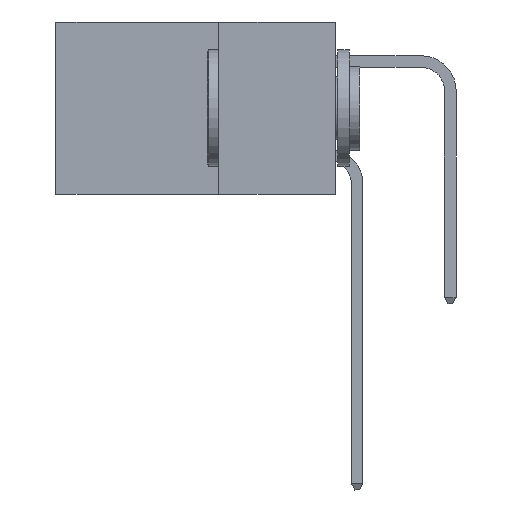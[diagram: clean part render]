
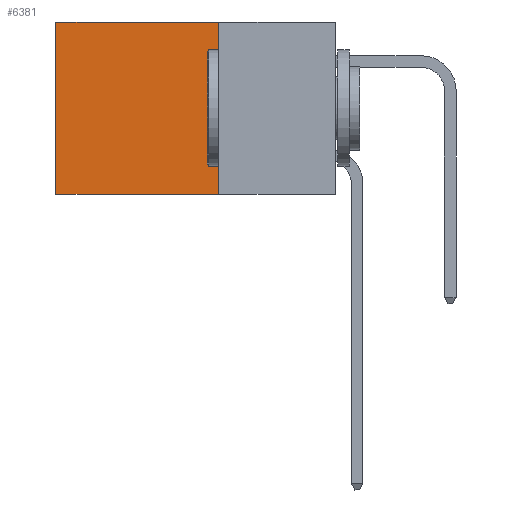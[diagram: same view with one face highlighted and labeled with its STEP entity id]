
A CAD part, left-side view. The second image highlights one B-rep face of the part: STEP entity #6381.
In plain terms, the highlighted planar face has unit normal (-1, 0, 0).
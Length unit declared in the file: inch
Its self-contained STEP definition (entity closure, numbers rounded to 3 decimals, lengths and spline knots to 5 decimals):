
#3 = CARTESIAN_POINT ( 'NONE',  ( 0.2875, 0.6, 0. ) ) ;
#42 = LINE ( 'NONE', #8670, #1972 ) ;
#457 = DIRECTION ( 'NONE',  ( 0., 1., 0. ) ) ;
#927 = ORIENTED_EDGE ( 'NONE', *, *, #6193, .F. ) ;
#1225 = LINE ( 'NONE', #3, #19461 ) ;
#1631 = VERTEX_POINT ( 'NONE', #9427 ) ;
#1972 = VECTOR ( 'NONE', #19196, 39.37008 ) ;
#2108 = LINE ( 'NONE', #10840, #22839 ) ;
#2180 = EDGE_CURVE ( 'NONE', #3280, #7720, #42, .T. ) ;
#3280 = VERTEX_POINT ( 'NONE', #22002 ) ;
#4042 = DIRECTION ( 'NONE',  ( 0., 0., -1. ) ) ;
#4323 = CARTESIAN_POINT ( 'NONE',  ( 0.2875, 0.25, -0.37 ) ) ;
#5308 = DIRECTION ( 'NONE',  ( 0., 0., -1. ) ) ;
#5985 = CARTESIAN_POINT ( 'NONE',  ( 0.2875, 0.6, 0. ) ) ;
#6193 = EDGE_CURVE ( 'NONE', #3280, #9025, #2108, .T. ) ;
#6381 = ADVANCED_FACE ( 'NONE', ( #9221 ), #22320, .F. ) ;
#6925 = ORIENTED_EDGE ( 'NONE', *, *, #21769, .T. ) ;
#7072 = EDGE_CURVE ( 'NONE', #9025, #1631, #20587, .T. ) ;
#7402 = ORIENTED_EDGE ( 'NONE', *, *, #2180, .T. ) ;
#7720 = VERTEX_POINT ( 'NONE', #5985 ) ;
#8670 = CARTESIAN_POINT ( 'NONE',  ( 0.2875, 0.25, 0. ) ) ;
#9025 = VERTEX_POINT ( 'NONE', #15469 ) ;
#9221 = FACE_OUTER_BOUND ( 'NONE', #13423, .T. ) ;
#9229 = VECTOR ( 'NONE', #457, 39.37008 ) ;
#9427 = CARTESIAN_POINT ( 'NONE',  ( 0.2875, 0.6, -0.37 ) ) ;
#9496 = AXIS2_PLACEMENT_3D ( 'NONE', #22469, #10516, #14103 ) ;
#10516 = DIRECTION ( 'NONE',  ( 1., 0., 0. ) ) ;
#10840 = CARTESIAN_POINT ( 'NONE',  ( 0.2875, 0.25, 0. ) ) ;
#13423 = EDGE_LOOP ( 'NONE', ( #6925, #21875, #927, #7402 ) ) ;
#14103 = DIRECTION ( 'NONE',  ( 0., 0., -1. ) ) ;
#15469 = CARTESIAN_POINT ( 'NONE',  ( 0.2875, 0.25, -0.37 ) ) ;
#19196 = DIRECTION ( 'NONE',  ( 0., 1., 0. ) ) ;
#19461 = VECTOR ( 'NONE', #5308, 39.37008 ) ;
#20587 = LINE ( 'NONE', #4323, #9229 ) ;
#21769 = EDGE_CURVE ( 'NONE', #7720, #1631, #1225, .T. ) ;
#21875 = ORIENTED_EDGE ( 'NONE', *, *, #7072, .F. ) ;
#22002 = CARTESIAN_POINT ( 'NONE',  ( 0.2875, 0.25, 0. ) ) ;
#22320 = PLANE ( 'NONE',  #9496 ) ;
#22469 = CARTESIAN_POINT ( 'NONE',  ( 0.2875, 0.25, 0. ) ) ;
#22839 = VECTOR ( 'NONE', #4042, 39.37008 ) ;
